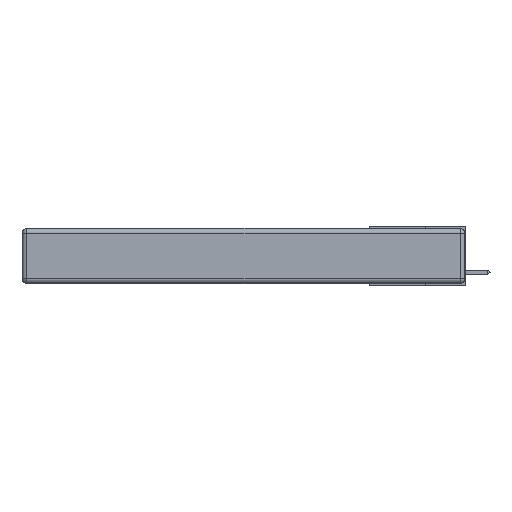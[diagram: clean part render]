
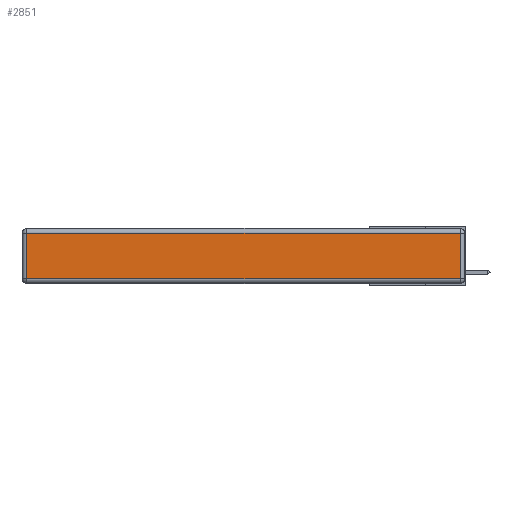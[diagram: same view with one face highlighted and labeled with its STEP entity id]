
A CAD part, left-side view. The second image highlights one B-rep face of the part: STEP entity #2851.
In plain terms, the highlighted planar face has unit normal (-1, 0, 0).
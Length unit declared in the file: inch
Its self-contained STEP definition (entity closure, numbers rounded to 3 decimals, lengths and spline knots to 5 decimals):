
#2092 = CARTESIAN_POINT ( 'NONE',  ( 0., 0., -0.343 ) ) ;
#2372 = DIRECTION ( 'NONE',  ( 0., 0., -1. ) ) ;
#2851 = ADVANCED_FACE ( 'NONE', ( #3200 ), #25699, .T. ) ;
#3200 = FACE_OUTER_BOUND ( 'NONE', #17971, .T. ) ;
#3718 = LINE ( 'NONE', #21080, #25251 ) ;
#4058 = ORIENTED_EDGE ( 'NONE', *, *, #14980, .T. ) ;
#4265 = DIRECTION ( 'NONE',  ( -1., 0., 0. ) ) ;
#4724 = CARTESIAN_POINT ( 'NONE',  ( 0., 0.03, -0.03 ) ) ;
#5940 = CARTESIAN_POINT ( 'NONE',  ( 0., 0.03, -0.343 ) ) ;
#7258 = LINE ( 'NONE', #12499, #22757 ) ;
#7721 = VERTEX_POINT ( 'NONE', #4724 ) ;
#8173 = DIRECTION ( 'NONE',  ( 0., -1., 0. ) ) ;
#9283 = ORIENTED_EDGE ( 'NONE', *, *, #13467, .T. ) ;
#9320 = VECTOR ( 'NONE', #12050, 39.37008 ) ;
#9516 = AXIS2_PLACEMENT_3D ( 'NONE', #2092, #4265, #17074 ) ;
#9542 = CARTESIAN_POINT ( 'NONE',  ( 0., 0.03, -0.313 ) ) ;
#10256 = DIRECTION ( 'NONE',  ( 0., 1., 0. ) ) ;
#10662 = LINE ( 'NONE', #5940, #9320 ) ;
#11073 = VERTEX_POINT ( 'NONE', #11684 ) ;
#11684 = CARTESIAN_POINT ( 'NONE',  ( 0., 2.72, -0.313 ) ) ;
#12050 = DIRECTION ( 'NONE',  ( 0., 0., 1. ) ) ;
#12079 = ORIENTED_EDGE ( 'NONE', *, *, #17073, .T. ) ;
#12499 = CARTESIAN_POINT ( 'NONE',  ( 0., 2.75, -0.03 ) ) ;
#13380 = CARTESIAN_POINT ( 'NONE',  ( 0., 2.72, -0.343 ) ) ;
#13467 = EDGE_CURVE ( 'NONE', #15029, #11073, #26021, .T. ) ;
#14749 = CARTESIAN_POINT ( 'NONE',  ( 0., 2.72, -0.03 ) ) ;
#14980 = EDGE_CURVE ( 'NONE', #11073, #23455, #3718, .T. ) ;
#15029 = VERTEX_POINT ( 'NONE', #14749 ) ;
#16643 = EDGE_CURVE ( 'NONE', #23455, #7721, #10662, .T. ) ;
#17073 = EDGE_CURVE ( 'NONE', #7721, #15029, #7258, .T. ) ;
#17074 = DIRECTION ( 'NONE',  ( 0., 0., 1. ) ) ;
#17971 = EDGE_LOOP ( 'NONE', ( #4058, #22521, #12079, #9283 ) ) ;
#20312 = VECTOR ( 'NONE', #2372, 39.37008 ) ;
#21080 = CARTESIAN_POINT ( 'NONE',  ( 0., 0., -0.313 ) ) ;
#22521 = ORIENTED_EDGE ( 'NONE', *, *, #16643, .T. ) ;
#22757 = VECTOR ( 'NONE', #10256, 39.37008 ) ;
#23455 = VERTEX_POINT ( 'NONE', #9542 ) ;
#25251 = VECTOR ( 'NONE', #8173, 39.37008 ) ;
#25699 = PLANE ( 'NONE',  #9516 ) ;
#26021 = LINE ( 'NONE', #13380, #20312 ) ;
